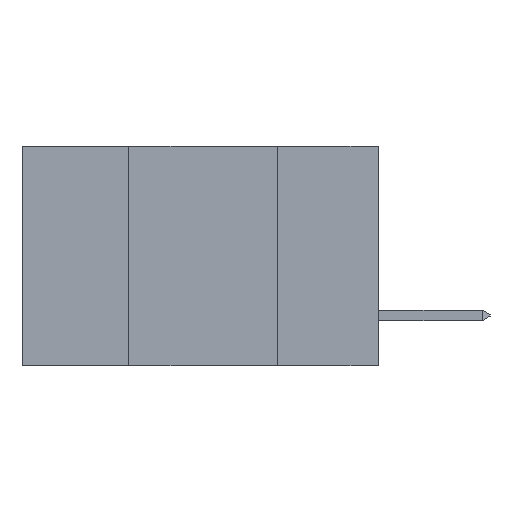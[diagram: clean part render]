
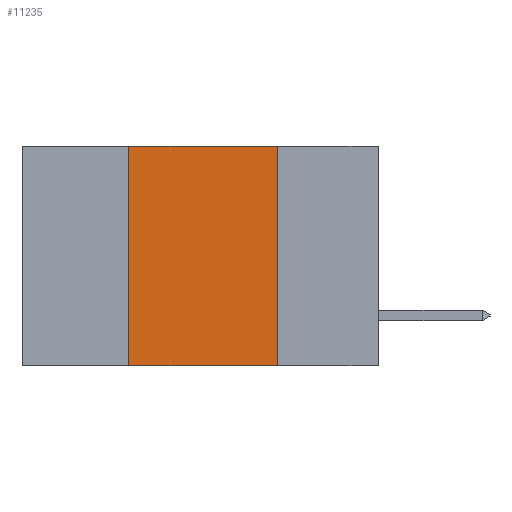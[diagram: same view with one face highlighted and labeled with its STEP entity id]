
A CAD part, left-side view. The second image highlights one B-rep face of the part: STEP entity #11235.
In plain terms, the highlighted planar face has unit normal (-1, 0, 0).
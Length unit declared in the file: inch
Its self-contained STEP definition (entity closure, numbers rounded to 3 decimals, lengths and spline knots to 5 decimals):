
#933 = CARTESIAN_POINT ( 'NONE',  ( 0., 0.17, 0. ) ) ;
#958 = VECTOR ( 'NONE', #8062, 39.37008 ) ;
#1173 = CARTESIAN_POINT ( 'NONE',  ( 0., 0.17, -0.37 ) ) ;
#1590 = VECTOR ( 'NONE', #16695, 39.37008 ) ;
#2285 = CARTESIAN_POINT ( 'NONE',  ( 0., 0.6, -0.37 ) ) ;
#2741 = VECTOR ( 'NONE', #6302, 39.37008 ) ;
#3178 = EDGE_LOOP ( 'NONE', ( #15026, #14636, #14850, #15031 ) ) ;
#3202 = LINE ( 'NONE', #16348, #2741 ) ;
#3645 = CARTESIAN_POINT ( 'NONE',  ( 0., 0.42, -0.37 ) ) ;
#4160 = PLANE ( 'NONE',  #15901 ) ;
#5614 = CARTESIAN_POINT ( 'NONE',  ( 0., 0.6, 0. ) ) ;
#6051 = CARTESIAN_POINT ( 'NONE',  ( 0., 0.42, 0. ) ) ;
#6302 = DIRECTION ( 'NONE',  ( 0., 0., -1. ) ) ;
#6452 = VECTOR ( 'NONE', #12123, 39.37008 ) ;
#7582 = CARTESIAN_POINT ( 'NONE',  ( 0., 0.42, -0.37 ) ) ;
#7832 = VERTEX_POINT ( 'NONE', #1173 ) ;
#8062 = DIRECTION ( 'NONE',  ( 0., 0., 1. ) ) ;
#8600 = DIRECTION ( 'NONE',  ( 0., 0., -1. ) ) ;
#8759 = FACE_OUTER_BOUND ( 'NONE', #3178, .T. ) ;
#9655 = EDGE_CURVE ( 'NONE', #10334, #18059, #14169, .T. ) ;
#10334 = VERTEX_POINT ( 'NONE', #6051 ) ;
#11235 = ADVANCED_FACE ( 'NONE', ( #8759 ), #4160, .F. ) ;
#11559 = EDGE_CURVE ( 'NONE', #18059, #7832, #3202, .T. ) ;
#12123 = DIRECTION ( 'NONE',  ( 0., -1., 0. ) ) ;
#12180 = VERTEX_POINT ( 'NONE', #7582 ) ;
#12293 = CARTESIAN_POINT ( 'NONE',  ( 0., 0.6, 0. ) ) ;
#13861 = EDGE_CURVE ( 'NONE', #12180, #7832, #17362, .T. ) ;
#14169 = LINE ( 'NONE', #12293, #6452 ) ;
#14636 = ORIENTED_EDGE ( 'NONE', *, *, #9655, .F. ) ;
#14850 = ORIENTED_EDGE ( 'NONE', *, *, #17522, .F. ) ;
#15026 = ORIENTED_EDGE ( 'NONE', *, *, #11559, .F. ) ;
#15031 = ORIENTED_EDGE ( 'NONE', *, *, #13861, .T. ) ;
#15901 = AXIS2_PLACEMENT_3D ( 'NONE', #5614, #17068, #8600 ) ;
#15982 = LINE ( 'NONE', #3645, #958 ) ;
#16348 = CARTESIAN_POINT ( 'NONE',  ( 0., 0.17, -0.37 ) ) ;
#16695 = DIRECTION ( 'NONE',  ( 0., -1., 0. ) ) ;
#17068 = DIRECTION ( 'NONE',  ( 1., 0., 0. ) ) ;
#17362 = LINE ( 'NONE', #2285, #1590 ) ;
#17522 = EDGE_CURVE ( 'NONE', #12180, #10334, #15982, .T. ) ;
#18059 = VERTEX_POINT ( 'NONE', #933 ) ;
